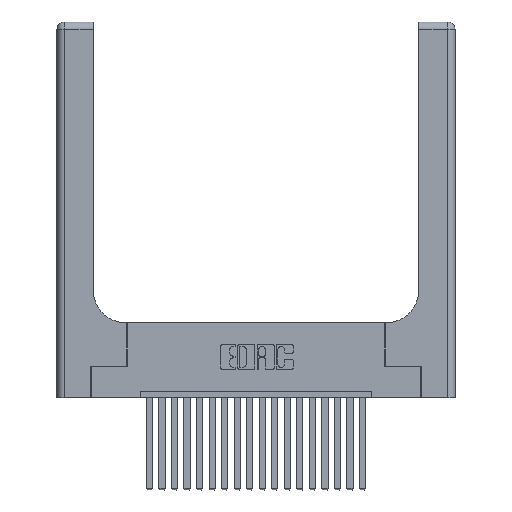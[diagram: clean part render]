
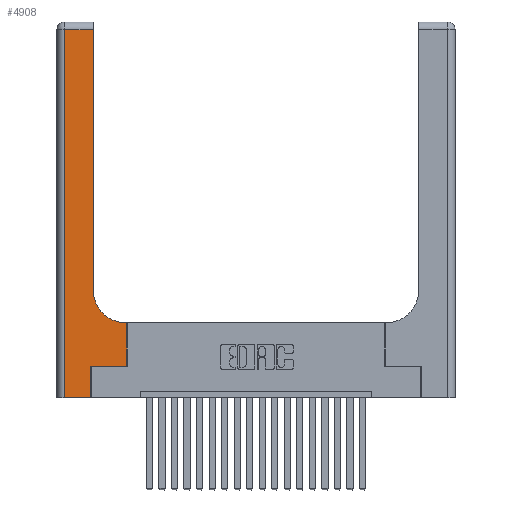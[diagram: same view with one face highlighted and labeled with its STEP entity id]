
A CAD part, top view. The second image highlights one B-rep face of the part: STEP entity #4908.
In plain terms, the highlighted planar face has unit normal (0, 0, 1).
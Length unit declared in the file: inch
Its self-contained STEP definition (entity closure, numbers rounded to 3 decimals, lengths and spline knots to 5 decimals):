
#588 = VECTOR ( 'NONE', #12995, 39.37008 ) ;
#948 = VECTOR ( 'NONE', #21763, 39.37008 ) ;
#1206 = DIRECTION ( 'NONE',  ( 1., 0., 0. ) ) ;
#1371 = CIRCLE ( 'NONE', #9434, 0.25 ) ;
#1433 = ORIENTED_EDGE ( 'NONE', *, *, #4673, .T. ) ;
#1557 = ORIENTED_EDGE ( 'NONE', *, *, #15141, .T. ) ;
#1996 = CARTESIAN_POINT ( 'NONE',  ( 0.06, 3., 0.37 ) ) ;
#2477 = VERTEX_POINT ( 'NONE', #19795 ) ;
#2669 = EDGE_CURVE ( 'NONE', #16303, #15328, #9850, .T. ) ;
#2769 = VECTOR ( 'NONE', #5534, 39.37008 ) ;
#3224 = CARTESIAN_POINT ( 'NONE',  ( 0.269, 0., 0.37 ) ) ;
#3329 = CARTESIAN_POINT ( 'NONE',  ( 0.2915, 3., 0.37 ) ) ;
#3750 = VECTOR ( 'NONE', #15962, 39.37008 ) ;
#4031 = VERTEX_POINT ( 'NONE', #10714 ) ;
#4673 = EDGE_CURVE ( 'NONE', #21334, #2477, #14770, .T. ) ;
#4831 = VERTEX_POINT ( 'NONE', #17096 ) ;
#4908 = ADVANCED_FACE ( 'NONE', ( #21057 ), #12332, .F. ) ;
#5200 = VECTOR ( 'NONE', #8635, 39.37008 ) ;
#5534 = DIRECTION ( 'NONE',  ( 0., -1., 0. ) ) ;
#5592 = DIRECTION ( 'NONE',  ( 0., 0., -1. ) ) ;
#6282 = EDGE_CURVE ( 'NONE', #10564, #8411, #21534, .T. ) ;
#6375 = LINE ( 'NONE', #17479, #11417 ) ;
#6485 = EDGE_LOOP ( 'NONE', ( #1433, #20200, #10646, #13269, #21549, #14186, #10910, #1557, #8647 ) ) ;
#6827 = CARTESIAN_POINT ( 'NONE',  ( 0.269, 0., 0.37 ) ) ;
#6916 = DIRECTION ( 'NONE',  ( 0., 1., 0. ) ) ;
#7481 = EDGE_CURVE ( 'NONE', #8411, #4031, #6375, .T. ) ;
#8411 = VERTEX_POINT ( 'NONE', #19960 ) ;
#8540 = EDGE_CURVE ( 'NONE', #2477, #16303, #9504, .T. ) ;
#8635 = DIRECTION ( 'NONE',  ( -1., 0., 0. ) ) ;
#8647 = ORIENTED_EDGE ( 'NONE', *, *, #13959, .T. ) ;
#8996 = DIRECTION ( 'NONE',  ( -1., 0., 0. ) ) ;
#9434 = AXIS2_PLACEMENT_3D ( 'NONE', #19554, #21402, #1206 ) ;
#9504 = LINE ( 'NONE', #18003, #588 ) ;
#9709 = LINE ( 'NONE', #20480, #5200 ) ;
#9850 = LINE ( 'NONE', #1996, #2769 ) ;
#10277 = DIRECTION ( 'NONE',  ( 1., 0., 0. ) ) ;
#10564 = VERTEX_POINT ( 'NONE', #10867 ) ;
#10646 = ORIENTED_EDGE ( 'NONE', *, *, #2669, .T. ) ;
#10657 = LINE ( 'NONE', #3224, #948 ) ;
#10714 = CARTESIAN_POINT ( 'NONE',  ( 0.5585, 0.6, 0.37 ) ) ;
#10867 = CARTESIAN_POINT ( 'NONE',  ( 0.269, 0.25, 0.37 ) ) ;
#10910 = ORIENTED_EDGE ( 'NONE', *, *, #7481, .T. ) ;
#11417 = VECTOR ( 'NONE', #20730, 39.37008 ) ;
#12332 = PLANE ( 'NONE',  #21171 ) ;
#12995 = DIRECTION ( 'NONE',  ( -1., 0., 0. ) ) ;
#13269 = ORIENTED_EDGE ( 'NONE', *, *, #19326, .T. ) ;
#13324 = CARTESIAN_POINT ( 'NONE',  ( 0.2915, 0.85, 0.37 ) ) ;
#13959 = EDGE_CURVE ( 'NONE', #4831, #21334, #1371, .T. ) ;
#14186 = ORIENTED_EDGE ( 'NONE', *, *, #6282, .T. ) ;
#14770 = LINE ( 'NONE', #3329, #20802 ) ;
#15141 = EDGE_CURVE ( 'NONE', #4031, #4831, #9709, .T. ) ;
#15292 = CARTESIAN_POINT ( 'NONE',  ( 0.269, 0.25, 0.37 ) ) ;
#15328 = VERTEX_POINT ( 'NONE', #21097 ) ;
#15744 = CARTESIAN_POINT ( 'NONE',  ( 0., 0., 0.37 ) ) ;
#15962 = DIRECTION ( 'NONE',  ( 1., 0., 0. ) ) ;
#16303 = VERTEX_POINT ( 'NONE', #19119 ) ;
#16397 = LINE ( 'NONE', #15744, #3750 ) ;
#17096 = CARTESIAN_POINT ( 'NONE',  ( 0.5415, 0.6, 0.37 ) ) ;
#17479 = CARTESIAN_POINT ( 'NONE',  ( 0.5585, 0.25, 0.37 ) ) ;
#17950 = EDGE_CURVE ( 'NONE', #19021, #10564, #10657, .T. ) ;
#18003 = CARTESIAN_POINT ( 'NONE',  ( 0., 2.94, 0.37 ) ) ;
#19021 = VERTEX_POINT ( 'NONE', #6827 ) ;
#19066 = CARTESIAN_POINT ( 'NONE',  ( 0., 3., 0.37 ) ) ;
#19119 = CARTESIAN_POINT ( 'NONE',  ( 0.06, 2.94, 0.37 ) ) ;
#19326 = EDGE_CURVE ( 'NONE', #15328, #19021, #16397, .T. ) ;
#19554 = CARTESIAN_POINT ( 'NONE',  ( 0.5415, 0.85, 0.37 ) ) ;
#19795 = CARTESIAN_POINT ( 'NONE',  ( 0.2915, 2.94, 0.37 ) ) ;
#19960 = CARTESIAN_POINT ( 'NONE',  ( 0.5585, 0.25, 0.37 ) ) ;
#20200 = ORIENTED_EDGE ( 'NONE', *, *, #8540, .T. ) ;
#20480 = CARTESIAN_POINT ( 'NONE',  ( 0.2915, 0.6, 0.37 ) ) ;
#20730 = DIRECTION ( 'NONE',  ( 0., 1., 0. ) ) ;
#20802 = VECTOR ( 'NONE', #6916, 39.37008 ) ;
#20992 = VECTOR ( 'NONE', #10277, 39.37008 ) ;
#21057 = FACE_OUTER_BOUND ( 'NONE', #6485, .T. ) ;
#21097 = CARTESIAN_POINT ( 'NONE',  ( 0.06, 0., 0.37 ) ) ;
#21171 = AXIS2_PLACEMENT_3D ( 'NONE', #19066, #5592, #8996 ) ;
#21334 = VERTEX_POINT ( 'NONE', #13324 ) ;
#21402 = DIRECTION ( 'NONE',  ( 0., 0., -1. ) ) ;
#21534 = LINE ( 'NONE', #15292, #20992 ) ;
#21549 = ORIENTED_EDGE ( 'NONE', *, *, #17950, .T. ) ;
#21763 = DIRECTION ( 'NONE',  ( 0., 1., 0. ) ) ;
